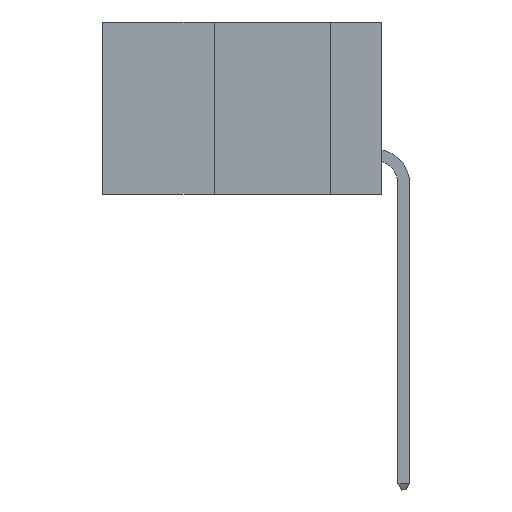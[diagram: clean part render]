
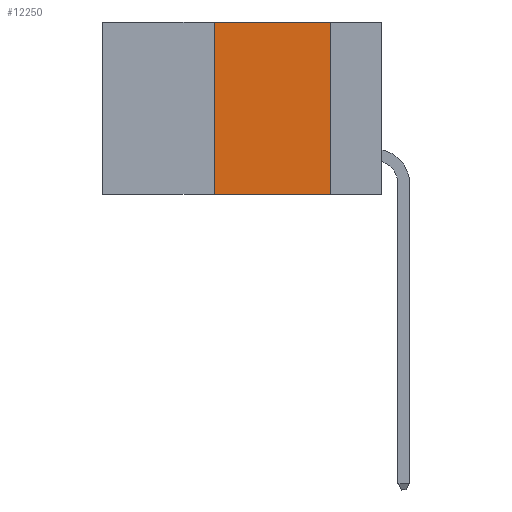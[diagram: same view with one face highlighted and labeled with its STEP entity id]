
A CAD part, left-side view. The second image highlights one B-rep face of the part: STEP entity #12250.
In plain terms, the highlighted planar face has unit normal (-1, 0, 0).
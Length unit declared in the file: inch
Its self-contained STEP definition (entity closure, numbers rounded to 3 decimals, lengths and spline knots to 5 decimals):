
#216 = CARTESIAN_POINT ( 'NONE',  ( 0., 0.6, 0. ) ) ;
#1710 = VERTEX_POINT ( 'NONE', #18206 ) ;
#2905 = VERTEX_POINT ( 'NONE', #19097 ) ;
#3362 = DIRECTION ( 'NONE',  ( 0., -1., 0. ) ) ;
#3651 = EDGE_LOOP ( 'NONE', ( #5770, #14953, #14194, #8021 ) ) ;
#5770 = ORIENTED_EDGE ( 'NONE', *, *, #17531, .F. ) ;
#5837 = VECTOR ( 'NONE', #20970, 39.37008 ) ;
#6208 = DIRECTION ( 'NONE',  ( 0., 0., -1. ) ) ;
#6767 = DIRECTION ( 'NONE',  ( 0., 0., 1. ) ) ;
#8021 = ORIENTED_EDGE ( 'NONE', *, *, #22555, .T. ) ;
#8517 = AXIS2_PLACEMENT_3D ( 'NONE', #10236, #24931, #6208 ) ;
#9685 = VECTOR ( 'NONE', #3362, 39.37008 ) ;
#10236 = CARTESIAN_POINT ( 'NONE',  ( 0., 0.6, 0. ) ) ;
#10328 = CARTESIAN_POINT ( 'NONE',  ( 0., 0.11, 0. ) ) ;
#10925 = CARTESIAN_POINT ( 'NONE',  ( 0., 0.36, 0. ) ) ;
#12250 = ADVANCED_FACE ( 'NONE', ( #19615 ), #18568, .F. ) ;
#13615 = CARTESIAN_POINT ( 'NONE',  ( 0., 0.6, -0.37 ) ) ;
#14194 = ORIENTED_EDGE ( 'NONE', *, *, #18767, .F. ) ;
#14474 = DIRECTION ( 'NONE',  ( 0., 0., -1. ) ) ;
#14953 = ORIENTED_EDGE ( 'NONE', *, *, #22774, .F. ) ;
#15104 = LINE ( 'NONE', #24895, #26474 ) ;
#15692 = LINE ( 'NONE', #10925, #24772 ) ;
#15871 = CARTESIAN_POINT ( 'NONE',  ( 0., 0.36, 0. ) ) ;
#17050 = VERTEX_POINT ( 'NONE', #10328 ) ;
#17531 = EDGE_CURVE ( 'NONE', #17050, #2905, #15104, .T. ) ;
#18206 = CARTESIAN_POINT ( 'NONE',  ( 0., 0.36, -0.37 ) ) ;
#18568 = PLANE ( 'NONE',  #8517 ) ;
#18767 = EDGE_CURVE ( 'NONE', #1710, #20880, #15692, .T. ) ;
#19097 = CARTESIAN_POINT ( 'NONE',  ( 0., 0.11, -0.37 ) ) ;
#19615 = FACE_OUTER_BOUND ( 'NONE', #3651, .T. ) ;
#20880 = VERTEX_POINT ( 'NONE', #15871 ) ;
#20970 = DIRECTION ( 'NONE',  ( 0., -1., 0. ) ) ;
#22555 = EDGE_CURVE ( 'NONE', #1710, #2905, #23969, .T. ) ;
#22774 = EDGE_CURVE ( 'NONE', #20880, #17050, #23282, .T. ) ;
#23282 = LINE ( 'NONE', #216, #5837 ) ;
#23969 = LINE ( 'NONE', #13615, #9685 ) ;
#24772 = VECTOR ( 'NONE', #6767, 39.37008 ) ;
#24895 = CARTESIAN_POINT ( 'NONE',  ( 0., 0.11, 0. ) ) ;
#24931 = DIRECTION ( 'NONE',  ( 1., 0., 0. ) ) ;
#26474 = VECTOR ( 'NONE', #14474, 39.37008 ) ;
